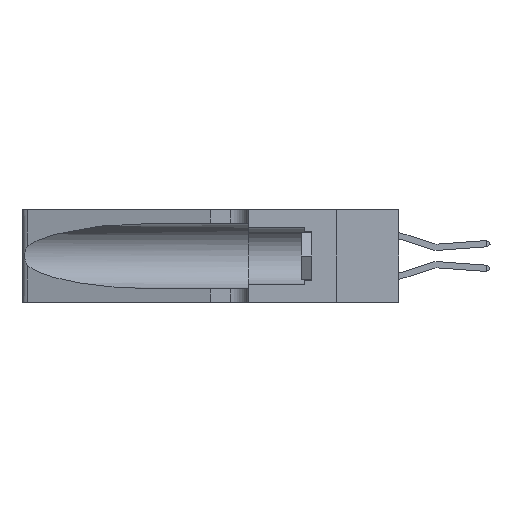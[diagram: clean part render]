
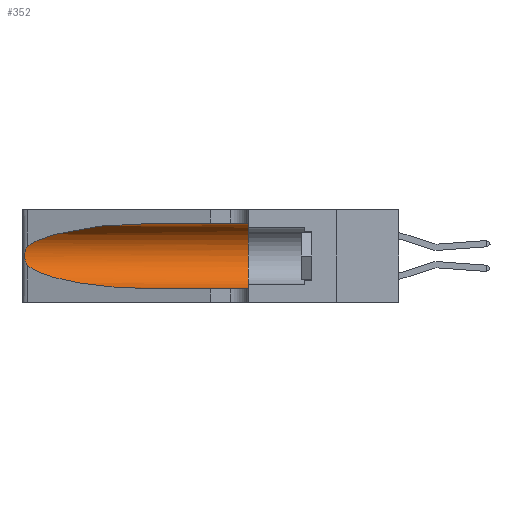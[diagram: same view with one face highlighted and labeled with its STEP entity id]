
A CAD part, left-side view. The second image highlights one B-rep face of the part: STEP entity #352.
In plain terms, the highlighted cylindrical face has radius 3.308 mm (diameter 6.617 mm), a partial arc.
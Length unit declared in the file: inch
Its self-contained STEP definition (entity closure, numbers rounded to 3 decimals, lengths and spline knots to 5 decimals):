
#352 = ADVANCED_FACE ( 'NONE', ( #2092 ), #22338, .F. ) ;
#685 = CARTESIAN_POINT ( 'NONE',  ( 0.25487, 1.22718, 0.14631 ) ) ;
#2092 = FACE_OUTER_BOUND ( 'NONE', #12572, .T. ) ;
#2732 = EDGE_CURVE ( 'NONE', #16739, #14965, #28310, .T. ) ;
#3265 = CARTESIAN_POINT ( 'NONE',  ( 0.25639, 1.23184, 0.21858 ) ) ;
#5495 = VERTEX_POINT ( 'NONE', #17457 ) ;
#5709 = CARTESIAN_POINT ( 'NONE',  ( 0.25487, 1.22718, 0.22369 ) ) ;
#5973 = CARTESIAN_POINT ( 'NONE',  ( 0.25854, 1.2359, 0.20912 ) ) ;
#6142 = CARTESIAN_POINT ( 'NONE',  ( 0.1305, 0.35, 0.05475 ) ) ;
#6580 = ORIENTED_EDGE ( 'NONE', *, *, #16927, .T. ) ;
#7004 = AXIS2_PLACEMENT_3D ( 'NONE', #22257, #18501, #24990 ) ;
#7465 = VECTOR ( 'NONE', #30740, 39.37008 ) ;
#8143 = CARTESIAN_POINT ( 'NONE',  ( 0.1305, 0.35, 0.31525 ) ) ;
#8661 = CARTESIAN_POINT ( 'NONE',  ( 0.26075, 1.23896, 0.19203 ) ) ;
#8977 = ORIENTED_EDGE ( 'NONE', *, *, #19216, .T. ) ;
#9716 = VERTEX_POINT ( 'NONE', #26693 ) ;
#10435 =( BOUNDED_CURVE ( )  B_SPLINE_CURVE ( 3, ( #16252, #23966, #21487, #5709 ),
 .UNSPECIFIED., .F., .T. ) 
 B_SPLINE_CURVE_WITH_KNOTS ( ( 4, 4 ),
 ( 1.5708, 2.84003 ),
 .UNSPECIFIED. ) 
 CURVE ( )  GEOMETRIC_REPRESENTATION_ITEM ( )  RATIONAL_B_SPLINE_CURVE ( ( 1., 0.87, 0.87, 1. ) ) 
 REPRESENTATION_ITEM ( '' )  );
#10626 = CARTESIAN_POINT ( 'NONE',  ( 0.1305, 0.72297, 0.05475 ) ) ;
#11246 = CARTESIAN_POINT ( 'NONE',  ( 0.25487, 1.22718, 0.22369 ) ) ;
#11359 = CARTESIAN_POINT ( 'NONE',  ( 0.26017, 1.23833, 0.17102 ) ) ;
#11675 = EDGE_CURVE ( 'NONE', #22017, #13805, #28046, .T. ) ;
#12104 = DIRECTION ( 'NONE',  ( 0., 1., 0. ) ) ;
#12572 = EDGE_LOOP ( 'NONE', ( #8977, #21102, #6580, #16038, #33789, #24482 ) ) ;
#12732 = CIRCLE ( 'NONE', #17178, 0.13025 ) ;
#13805 = VERTEX_POINT ( 'NONE', #6142 ) ;
#13992 = CARTESIAN_POINT ( 'NONE',  ( 0.25789, 1.23486, 0.15765 ) ) ;
#14965 = VERTEX_POINT ( 'NONE', #8143 ) ;
#15175 = CARTESIAN_POINT ( 'NONE',  ( 0.1305, 0.72297, 0.05475 ) ) ;
#16038 = ORIENTED_EDGE ( 'NONE', *, *, #11675, .T. ) ;
#16252 = CARTESIAN_POINT ( 'NONE',  ( 0.1305, 0.72297, 0.31525 ) ) ;
#16521 = B_SPLINE_CURVE_WITH_KNOTS ( 'NONE', 3,
 ( #11246, #24226, #3265, #21751, #5973, #24332, #8661, #26908, #11359, #29492, #13992, #32067, #16612, #685 ),
 .UNSPECIFIED., .F., .F.,
 ( 4, 2, 2, 2, 2, 2, 4 ),
 ( 0., 0.00027, 0.00053, 0.00107, 0.0016, 0.00187, 0.00214 ),
 .UNSPECIFIED. ) ;
#16612 = CARTESIAN_POINT ( 'NONE',  ( 0.25555, 1.22993, 0.14849 ) ) ;
#16739 = VERTEX_POINT ( 'NONE', #17737 ) ;
#16927 = EDGE_CURVE ( 'NONE', #5495, #22017, #22586, .T. ) ;
#17178 = AXIS2_PLACEMENT_3D ( 'NONE', #27621, #12104, #30223 ) ;
#17457 = CARTESIAN_POINT ( 'NONE',  ( 0.25487, 1.22718, 0.14631 ) ) ;
#17655 = CARTESIAN_POINT ( 'NONE',  ( 0.1305, 1.61858, 0.31525 ) ) ;
#17737 = CARTESIAN_POINT ( 'NONE',  ( 0.1305, 0.72297, 0.31525 ) ) ;
#18501 = DIRECTION ( 'NONE',  ( 0., -1., 0. ) ) ;
#18634 = EDGE_CURVE ( 'NONE', #9716, #5495, #16521, .T. ) ;
#19216 = EDGE_CURVE ( 'NONE', #16739, #9716, #10435, .T. ) ;
#21029 = CARTESIAN_POINT ( 'NONE',  ( 0.25487, 1.22718, 0.14631 ) ) ;
#21102 = ORIENTED_EDGE ( 'NONE', *, *, #18634, .T. ) ;
#21487 = CARTESIAN_POINT ( 'NONE',  ( 0.2373, 1.15595, 0.28018 ) ) ;
#21751 = CARTESIAN_POINT ( 'NONE',  ( 0.25787, 1.23484, 0.2124 ) ) ;
#22017 = VERTEX_POINT ( 'NONE', #15175 ) ;
#22257 = CARTESIAN_POINT ( 'NONE',  ( 0.1305, 1.61858, 0.185 ) ) ;
#22338 = CYLINDRICAL_SURFACE ( 'NONE', #7004, 0.13025 ) ;
#22586 =( BOUNDED_CURVE ( )  B_SPLINE_CURVE ( 3, ( #21029, #28688, #26209, #10626 ),
 .UNSPECIFIED., .F., .F. ) 
 B_SPLINE_CURVE_WITH_KNOTS ( ( 4, 4 ),
 ( 3.44316, 4.71239 ),
 .UNSPECIFIED. ) 
 CURVE ( )  GEOMETRIC_REPRESENTATION_ITEM ( )  RATIONAL_B_SPLINE_CURVE ( ( 1., 0.87, 0.87, 1. ) ) 
 REPRESENTATION_ITEM ( '' )  );
#23966 = CARTESIAN_POINT ( 'NONE',  ( 0.18966, 0.96281, 0.31525 ) ) ;
#24226 = CARTESIAN_POINT ( 'NONE',  ( 0.25555, 1.22994, 0.2215 ) ) ;
#24332 = CARTESIAN_POINT ( 'NONE',  ( 0.26018, 1.23835, 0.19895 ) ) ;
#24482 = ORIENTED_EDGE ( 'NONE', *, *, #2732, .F. ) ;
#24990 = DIRECTION ( 'NONE',  ( 0., 0., -1. ) ) ;
#26209 = CARTESIAN_POINT ( 'NONE',  ( 0.18966, 0.96281, 0.05475 ) ) ;
#26693 = CARTESIAN_POINT ( 'NONE',  ( 0.25487, 1.22718, 0.22369 ) ) ;
#26908 = CARTESIAN_POINT ( 'NONE',  ( 0.26075, 1.23896, 0.178 ) ) ;
#27214 = VECTOR ( 'NONE', #28996, 39.37008 ) ;
#27621 = CARTESIAN_POINT ( 'NONE',  ( 0.1305, 0.35, 0.185 ) ) ;
#28046 = LINE ( 'NONE', #31564, #27214 ) ;
#28310 = LINE ( 'NONE', #17655, #7465 ) ;
#28688 = CARTESIAN_POINT ( 'NONE',  ( 0.2373, 1.15595, 0.08982 ) ) ;
#28996 = DIRECTION ( 'NONE',  ( 0., -1., 0. ) ) ;
#29492 = CARTESIAN_POINT ( 'NONE',  ( 0.25856, 1.23593, 0.16098 ) ) ;
#29782 = EDGE_CURVE ( 'NONE', #14965, #13805, #12732, .T. ) ;
#30223 = DIRECTION ( 'NONE',  ( 0., 0., 1. ) ) ;
#30740 = DIRECTION ( 'NONE',  ( 0., -1., 0. ) ) ;
#31564 = CARTESIAN_POINT ( 'NONE',  ( 0.1305, 1.61858, 0.05475 ) ) ;
#32067 = CARTESIAN_POINT ( 'NONE',  ( 0.25639, 1.23186, 0.15144 ) ) ;
#33789 = ORIENTED_EDGE ( 'NONE', *, *, #29782, .F. ) ;
